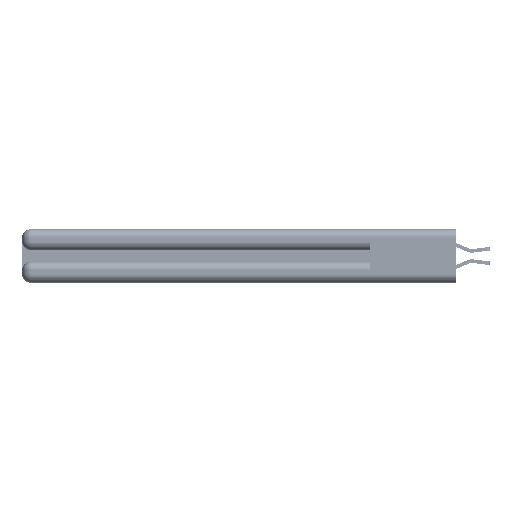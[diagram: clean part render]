
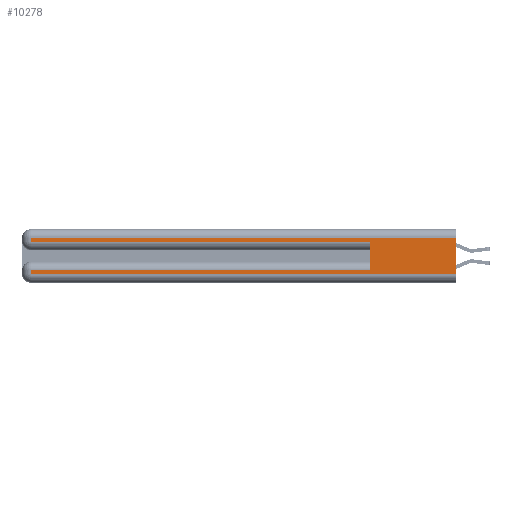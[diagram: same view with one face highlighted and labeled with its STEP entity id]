
A CAD part, left-side view. The second image highlights one B-rep face of the part: STEP entity #10278.
In plain terms, the highlighted planar face has unit normal (-1, 0, 0).
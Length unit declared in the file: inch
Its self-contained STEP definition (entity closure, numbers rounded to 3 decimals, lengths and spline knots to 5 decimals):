
#453 = DIRECTION ( 'NONE',  ( 0., -1., 0. ) ) ;
#1494 = EDGE_CURVE ( 'NONE', #30269, #30214, #48819, .T. ) ;
#1518 = LINE ( 'NONE', #20322, #12251 ) ;
#1915 = EDGE_CURVE ( 'NONE', #30269, #39832, #35635, .T. ) ;
#2108 = FACE_OUTER_BOUND ( 'NONE', #45524, .T. ) ;
#2671 = VECTOR ( 'NONE', #4522, 39.37008 ) ;
#3153 = CARTESIAN_POINT ( 'NONE',  ( 0., 0., 0.37 ) ) ;
#4522 = DIRECTION ( 'NONE',  ( 0., -1., 0. ) ) ;
#5226 = CARTESIAN_POINT ( 'NONE',  ( 0., 0.6, 0.285 ) ) ;
#6184 = VECTOR ( 'NONE', #453, 39.37008 ) ;
#6658 = EDGE_CURVE ( 'NONE', #45194, #39832, #15032, .T. ) ;
#6697 = DIRECTION ( 'NONE',  ( 0., 0., -1. ) ) ;
#6818 = DIRECTION ( 'NONE',  ( 0., 0., -1. ) ) ;
#7813 = EDGE_CURVE ( 'NONE', #51881, #35864, #24372, .T. ) ;
#8700 = PLANE ( 'NONE',  #11403 ) ;
#9592 = LINE ( 'NONE', #36215, #2671 ) ;
#10202 = EDGE_CURVE ( 'NONE', #51881, #16468, #1518, .T. ) ;
#10278 = ADVANCED_FACE ( 'NONE', ( #2108 ), #8700, .F. ) ;
#11403 = AXIS2_PLACEMENT_3D ( 'NONE', #49035, #37013, #24888 ) ;
#11798 = VECTOR ( 'NONE', #22973, 39.37008 ) ;
#12251 = VECTOR ( 'NONE', #16806, 39.37008 ) ;
#15032 = LINE ( 'NONE', #48546, #6184 ) ;
#16468 = VERTEX_POINT ( 'NONE', #48515 ) ;
#16806 = DIRECTION ( 'NONE',  ( 0., 1., 0. ) ) ;
#17553 = ORIENTED_EDGE ( 'NONE', *, *, #1494, .T. ) ;
#20322 = CARTESIAN_POINT ( 'NONE',  ( 0., 0., 0.085 ) ) ;
#20982 = VECTOR ( 'NONE', #37221, 39.37008 ) ;
#21244 = VERTEX_POINT ( 'NONE', #48274 ) ;
#21569 = LINE ( 'NONE', #33190, #20982 ) ;
#22973 = DIRECTION ( 'NONE',  ( 0., 0., 1. ) ) ;
#23269 = CARTESIAN_POINT ( 'NONE',  ( 0., 0., 0.31 ) ) ;
#23538 = ORIENTED_EDGE ( 'NONE', *, *, #33152, .T. ) ;
#24372 = LINE ( 'NONE', #43064, #11798 ) ;
#24888 = DIRECTION ( 'NONE',  ( 0., 0., -1. ) ) ;
#24934 = VECTOR ( 'NONE', #6697, 39.37008 ) ;
#28917 = ORIENTED_EDGE ( 'NONE', *, *, #6658, .T. ) ;
#30214 = VERTEX_POINT ( 'NONE', #51248 ) ;
#30269 = VERTEX_POINT ( 'NONE', #32221 ) ;
#31850 = ORIENTED_EDGE ( 'NONE', *, *, #1915, .F. ) ;
#31857 = LINE ( 'NONE', #34596, #43174 ) ;
#32221 = CARTESIAN_POINT ( 'NONE',  ( 0., 0., 0.31 ) ) ;
#32602 = DIRECTION ( 'NONE',  ( 0., 1., 0. ) ) ;
#33152 = EDGE_CURVE ( 'NONE', #30214, #21244, #31857, .T. ) ;
#33190 = CARTESIAN_POINT ( 'NONE',  ( 0., 2.94, 0.37 ) ) ;
#34596 = CARTESIAN_POINT ( 'NONE',  ( 0., 2.94, 0.37 ) ) ;
#35635 = LINE ( 'NONE', #3153, #24934 ) ;
#35864 = VERTEX_POINT ( 'NONE', #5226 ) ;
#36215 = CARTESIAN_POINT ( 'NONE',  ( 0., 0., 0.285 ) ) ;
#36587 = CARTESIAN_POINT ( 'NONE',  ( 0., 0., 0.06 ) ) ;
#37013 = DIRECTION ( 'NONE',  ( 1., 0., 0. ) ) ;
#37221 = DIRECTION ( 'NONE',  ( 0., 0., -1. ) ) ;
#37942 = ORIENTED_EDGE ( 'NONE', *, *, #7813, .F. ) ;
#38035 = VECTOR ( 'NONE', #32602, 39.37008 ) ;
#39311 = EDGE_CURVE ( 'NONE', #21244, #35864, #9592, .T. ) ;
#39384 = EDGE_CURVE ( 'NONE', #16468, #45194, #21569, .T. ) ;
#39832 = VERTEX_POINT ( 'NONE', #36587 ) ;
#41452 = ORIENTED_EDGE ( 'NONE', *, *, #39311, .T. ) ;
#42988 = ORIENTED_EDGE ( 'NONE', *, *, #39384, .T. ) ;
#43064 = CARTESIAN_POINT ( 'NONE',  ( 0., 0.6, 0.145 ) ) ;
#43174 = VECTOR ( 'NONE', #6818, 39.37008 ) ;
#45194 = VERTEX_POINT ( 'NONE', #46172 ) ;
#45524 = EDGE_LOOP ( 'NONE', ( #31850, #17553, #23538, #41452, #37942, #46777, #42988, #28917 ) ) ;
#46172 = CARTESIAN_POINT ( 'NONE',  ( 0., 2.94, 0.06 ) ) ;
#46644 = CARTESIAN_POINT ( 'NONE',  ( 0., 0.6, 0.085 ) ) ;
#46777 = ORIENTED_EDGE ( 'NONE', *, *, #10202, .T. ) ;
#48274 = CARTESIAN_POINT ( 'NONE',  ( 0., 2.94, 0.285 ) ) ;
#48515 = CARTESIAN_POINT ( 'NONE',  ( 0., 2.94, 0.085 ) ) ;
#48546 = CARTESIAN_POINT ( 'NONE',  ( 0., 0., 0.06 ) ) ;
#48819 = LINE ( 'NONE', #23269, #38035 ) ;
#49035 = CARTESIAN_POINT ( 'NONE',  ( 0., 0., 0.37 ) ) ;
#51248 = CARTESIAN_POINT ( 'NONE',  ( 0., 2.94, 0.31 ) ) ;
#51881 = VERTEX_POINT ( 'NONE', #46644 ) ;
